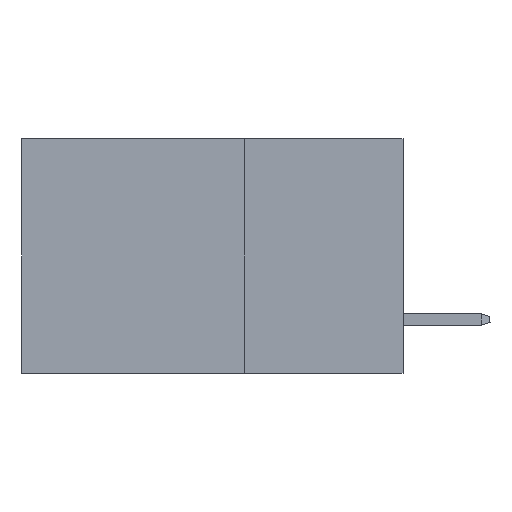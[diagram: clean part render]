
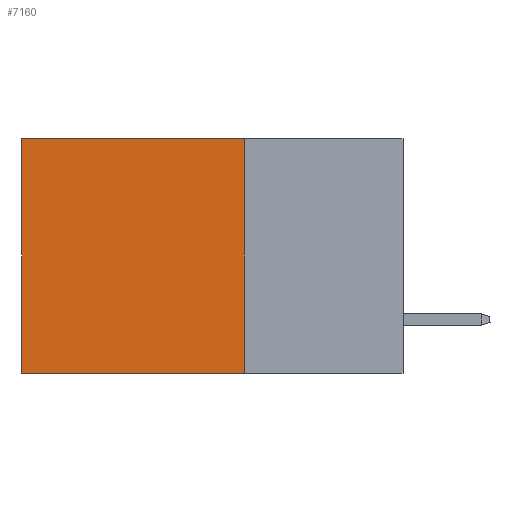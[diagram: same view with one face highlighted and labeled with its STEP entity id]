
A CAD part, left-side view. The second image highlights one B-rep face of the part: STEP entity #7160.
In plain terms, the highlighted planar face has unit normal (-1, 0, 0).
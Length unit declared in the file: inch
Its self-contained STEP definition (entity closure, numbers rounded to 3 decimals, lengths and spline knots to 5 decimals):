
#47 = EDGE_CURVE ( 'NONE', #37325, #34322, #2397, .T. ) ;
#509 = VECTOR ( 'NONE', #19825, 39.37008 ) ;
#2397 = LINE ( 'NONE', #22498, #509 ) ;
#2639 = CARTESIAN_POINT ( 'NONE',  ( 0.2875, 0.25, -0.37 ) ) ;
#3815 = DIRECTION ( 'NONE',  ( 0., 1., 0. ) ) ;
#6072 = VECTOR ( 'NONE', #3815, 39.37008 ) ;
#7160 = ADVANCED_FACE ( 'NONE', ( #27869 ), #17272, .F. ) ;
#8696 = AXIS2_PLACEMENT_3D ( 'NONE', #9967, #38469, #21020 ) ;
#9012 = CARTESIAN_POINT ( 'NONE',  ( 0.2875, 0.6, 0. ) ) ;
#9967 = CARTESIAN_POINT ( 'NONE',  ( 0.2875, 0.25, 0. ) ) ;
#11414 = CARTESIAN_POINT ( 'NONE',  ( 0.2875, 0.25, 0. ) ) ;
#12420 = ORIENTED_EDGE ( 'NONE', *, *, #26182, .F. ) ;
#17065 = CARTESIAN_POINT ( 'NONE',  ( 0.2875, 0.25, 0. ) ) ;
#17272 = PLANE ( 'NONE',  #8696 ) ;
#18140 = EDGE_LOOP ( 'NONE', ( #18884, #12420, #35993, #35696 ) ) ;
#18634 = LINE ( 'NONE', #40523, #6072 ) ;
#18884 = ORIENTED_EDGE ( 'NONE', *, *, #47, .T. ) ;
#19825 = DIRECTION ( 'NONE',  ( 0., 0., -1. ) ) ;
#21020 = DIRECTION ( 'NONE',  ( 0., 0., -1. ) ) ;
#22498 = CARTESIAN_POINT ( 'NONE',  ( 0.2875, 0.6, 0. ) ) ;
#23983 = CARTESIAN_POINT ( 'NONE',  ( 0.2875, 0.6, -0.37 ) ) ;
#24834 = DIRECTION ( 'NONE',  ( 0., 0., -1. ) ) ;
#26182 = EDGE_CURVE ( 'NONE', #45182, #34322, #41492, .T. ) ;
#26389 = EDGE_CURVE ( 'NONE', #37100, #37325, #18634, .T. ) ;
#27594 = DIRECTION ( 'NONE',  ( 0., 1., 0. ) ) ;
#27869 = FACE_OUTER_BOUND ( 'NONE', #18140, .T. ) ;
#28361 = LINE ( 'NONE', #11414, #33337 ) ;
#28859 = EDGE_CURVE ( 'NONE', #37100, #45182, #28361, .T. ) ;
#33150 = VECTOR ( 'NONE', #27594, 39.37008 ) ;
#33337 = VECTOR ( 'NONE', #24834, 39.37008 ) ;
#34322 = VERTEX_POINT ( 'NONE', #23983 ) ;
#35696 = ORIENTED_EDGE ( 'NONE', *, *, #26389, .T. ) ;
#35993 = ORIENTED_EDGE ( 'NONE', *, *, #28859, .F. ) ;
#37100 = VERTEX_POINT ( 'NONE', #17065 ) ;
#37325 = VERTEX_POINT ( 'NONE', #9012 ) ;
#38469 = DIRECTION ( 'NONE',  ( 1., 0., 0. ) ) ;
#40523 = CARTESIAN_POINT ( 'NONE',  ( 0.2875, 0.25, 0. ) ) ;
#41492 = LINE ( 'NONE', #2639, #33150 ) ;
#44399 = CARTESIAN_POINT ( 'NONE',  ( 0.2875, 0.25, -0.37 ) ) ;
#45182 = VERTEX_POINT ( 'NONE', #44399 ) ;
